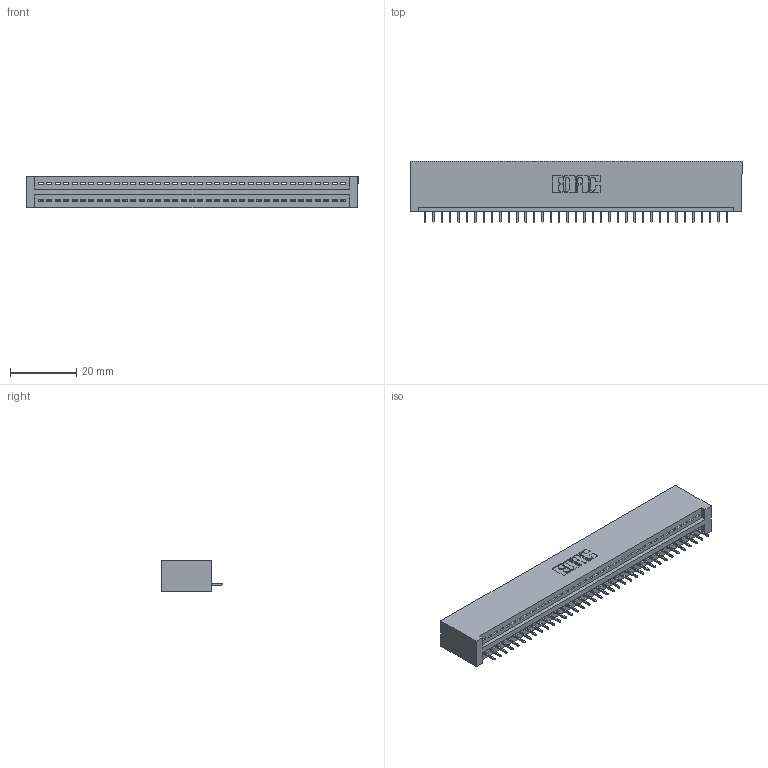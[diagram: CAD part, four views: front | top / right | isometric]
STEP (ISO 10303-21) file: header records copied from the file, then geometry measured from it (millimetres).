
FILE_DESCRIPTION (( 'STEP AP203' ), '1' );
FILE_NAME ('395-037-525-101.STEP', '2020-09-24T00:10:39', ( '' ), ( '' ), 'SwSTEP 2.0', 'SolidWorks 2020', '' );
FILE_SCHEMA (( 'CONFIG_CONTROL_DESIGN' ));
Length unit declared in the file: inch
Products named in the file (3): 345 Part_No Mounting Lugs; 345-292-001_345-293-125; 395-037-525-101
Assembly tree (38 placements, depth 2):
  395-037-525-101
    345 Part_No Mounting Lugs
    345-292-001_345-293-125  x37
Bounding box: 100.58 x 18.72 x 9.4 mm (x, y, z)
Volume: 9945.9 mm3; surface area: 12835.6 mm2
Topology: 38 solids, 38 shells, 2412 faces, 6977 edges, 4502 vertices
Faces by surface type: plane 1778, cylinder 634
Entity records: 28317 total; most frequent: CARTESIAN_POINT 4911, ORIENTED_EDGE 4882, DIRECTION 4291, EDGE_CURVE 2441, VECTOR 2173, LINE 2173, VERTEX_POINT 1622, AXIS2_PLACEMENT_3D 1059
